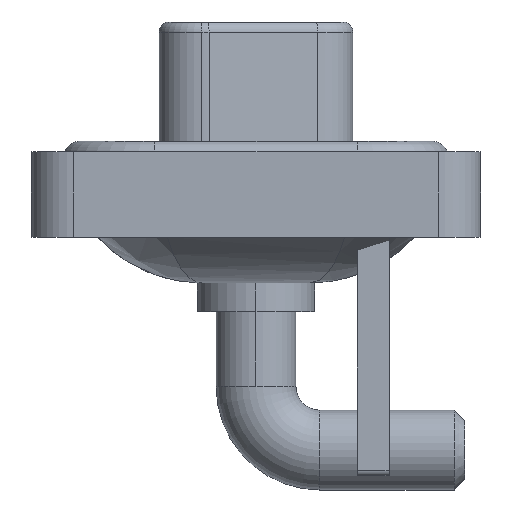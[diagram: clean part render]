
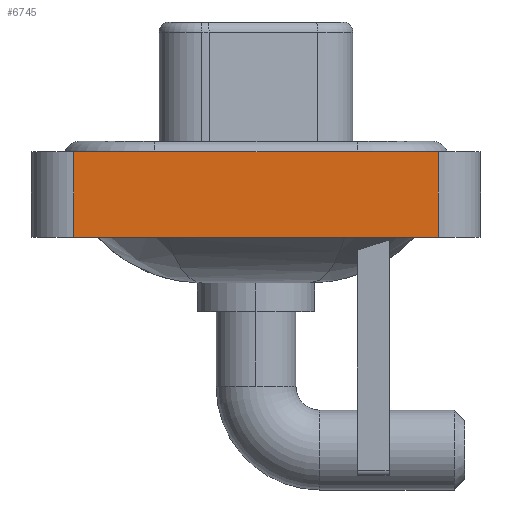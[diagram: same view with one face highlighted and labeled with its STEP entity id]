
A CAD part, left-side view. The second image highlights one B-rep face of the part: STEP entity #6745.
In plain terms, the highlighted planar face has unit normal (-1, 0, 0).
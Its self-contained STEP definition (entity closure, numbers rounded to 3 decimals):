
#712 = VECTOR ( 'NONE', #6245, 1000. ) ;
#964 = VECTOR ( 'NONE', #9229, 1000. ) ;
#1742 = CARTESIAN_POINT ( 'NONE',  ( -7.25, -8.55, -3.6 ) ) ;
#2265 = DIRECTION ( 'NONE',  ( -1., 0., 0. ) ) ;
#2988 = CARTESIAN_POINT ( 'NONE',  ( -7.25, -8.55, 0.4 ) ) ;
#3829 = CARTESIAN_POINT ( 'NONE',  ( -7.25, -8.55, 0.4 ) ) ;
#4208 = VECTOR ( 'NONE', #10212, 1000. ) ;
#4270 = LINE ( 'NONE', #2988, #4208 ) ;
#4739 = VECTOR ( 'NONE', #12191, 1000. ) ;
#4809 = ORIENTED_EDGE ( 'NONE', *, *, #8343, .T. ) ;
#5203 = LINE ( 'NONE', #7600, #712 ) ;
#5456 = LINE ( 'NONE', #10528, #964 ) ;
#6245 = DIRECTION ( 'NONE',  ( 0., 0., 1. ) ) ;
#6255 = CARTESIAN_POINT ( 'NONE',  ( -7.25, -8.55, -3.6 ) ) ;
#6434 = CARTESIAN_POINT ( 'NONE',  ( -7.25, 8.55, 0.4 ) ) ;
#6745 = ADVANCED_FACE ( 'NONE', ( #14266 ), #15635, .T. ) ;
#7600 = CARTESIAN_POINT ( 'NONE',  ( -7.25, 8.55, -3.6 ) ) ;
#8021 = EDGE_CURVE ( 'NONE', #12623, #10617, #4270, .T. ) ;
#8022 = ORIENTED_EDGE ( 'NONE', *, *, #9814, .T. ) ;
#8343 = EDGE_CURVE ( 'NONE', #8670, #12099, #10999, .T. ) ;
#8670 = VERTEX_POINT ( 'NONE', #13609 ) ;
#9229 = DIRECTION ( 'NONE',  ( 0., 0., 1. ) ) ;
#9769 = EDGE_LOOP ( 'NONE', ( #8022, #11876, #13014, #4809 ) ) ;
#9814 = EDGE_CURVE ( 'NONE', #12099, #10617, #5456, .T. ) ;
#10185 = EDGE_CURVE ( 'NONE', #8670, #12623, #5203, .T. ) ;
#10212 = DIRECTION ( 'NONE',  ( 0., -1., 0. ) ) ;
#10528 = CARTESIAN_POINT ( 'NONE',  ( -7.25, -8.55, -3.6 ) ) ;
#10617 = VERTEX_POINT ( 'NONE', #3829 ) ;
#10999 = LINE ( 'NONE', #6255, #4739 ) ;
#11722 = DIRECTION ( 'NONE',  ( 0., 0., 1. ) ) ;
#11876 = ORIENTED_EDGE ( 'NONE', *, *, #8021, .F. ) ;
#12099 = VERTEX_POINT ( 'NONE', #1742 ) ;
#12191 = DIRECTION ( 'NONE',  ( 0., -1., 0. ) ) ;
#12623 = VERTEX_POINT ( 'NONE', #6434 ) ;
#13014 = ORIENTED_EDGE ( 'NONE', *, *, #10185, .F. ) ;
#13609 = CARTESIAN_POINT ( 'NONE',  ( -7.25, 8.55, -3.6 ) ) ;
#14266 = FACE_OUTER_BOUND ( 'NONE', #9769, .T. ) ;
#14291 = AXIS2_PLACEMENT_3D ( 'NONE', #15462, #2265, #11722 ) ;
#15462 = CARTESIAN_POINT ( 'NONE',  ( -7.25, -8.55, -3.6 ) ) ;
#15635 = PLANE ( 'NONE',  #14291 ) ;
